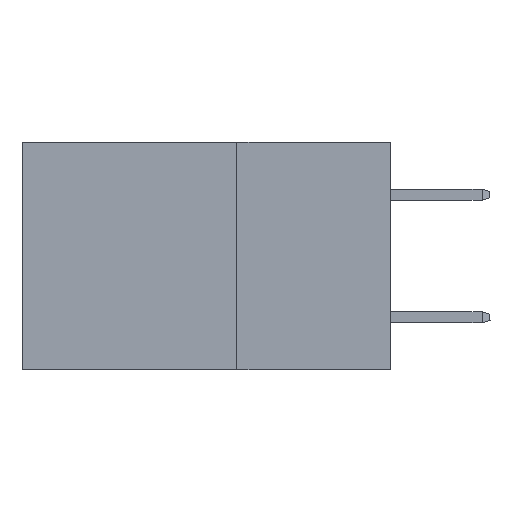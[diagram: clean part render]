
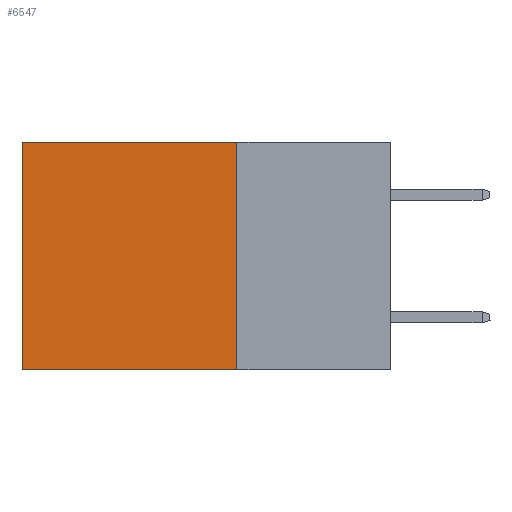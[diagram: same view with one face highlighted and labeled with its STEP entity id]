
A CAD part, left-side view. The second image highlights one B-rep face of the part: STEP entity #6547.
In plain terms, the highlighted planar face has unit normal (-1, 0, 0).
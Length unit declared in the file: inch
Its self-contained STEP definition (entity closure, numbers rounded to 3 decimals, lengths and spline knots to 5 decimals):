
#1896 = ORIENTED_EDGE ( 'NONE', *, *, #3113, .T. ) ;
#1969 = CARTESIAN_POINT ( 'NONE',  ( 0.2875, 0.25, 0. ) ) ;
#3113 = EDGE_CURVE ( 'NONE', #19517, #9737, #12800, .T. ) ;
#5117 = VERTEX_POINT ( 'NONE', #19602 ) ;
#5700 = ORIENTED_EDGE ( 'NONE', *, *, #10846, .F. ) ;
#6547 = ADVANCED_FACE ( 'NONE', ( #13472 ), #15747, .F. ) ;
#7428 = ORIENTED_EDGE ( 'NONE', *, *, #18647, .F. ) ;
#7660 = VECTOR ( 'NONE', #14456, 39.37008 ) ;
#8335 = AXIS2_PLACEMENT_3D ( 'NONE', #1969, #13083, #8481 ) ;
#8481 = DIRECTION ( 'NONE',  ( 0., 0., -1. ) ) ;
#8796 = VERTEX_POINT ( 'NONE', #15431 ) ;
#9110 = ORIENTED_EDGE ( 'NONE', *, *, #13517, .T. ) ;
#9220 = LINE ( 'NONE', #15464, #19022 ) ;
#9481 = CARTESIAN_POINT ( 'NONE',  ( 0.2875, 0.25, 0. ) ) ;
#9737 = VERTEX_POINT ( 'NONE', #13606 ) ;
#9877 = VECTOR ( 'NONE', #21310, 39.37008 ) ;
#10846 = EDGE_CURVE ( 'NONE', #19517, #8796, #18110, .T. ) ;
#12800 = LINE ( 'NONE', #21198, #21281 ) ;
#13083 = DIRECTION ( 'NONE',  ( 1., 0., 0. ) ) ;
#13472 = FACE_OUTER_BOUND ( 'NONE', #15023, .T. ) ;
#13517 = EDGE_CURVE ( 'NONE', #9737, #5117, #9220, .T. ) ;
#13606 = CARTESIAN_POINT ( 'NONE',  ( 0.2875, 0.6, 0. ) ) ;
#14306 = CARTESIAN_POINT ( 'NONE',  ( 0.2875, 0.25, -0.37 ) ) ;
#14392 = CARTESIAN_POINT ( 'NONE',  ( 0.2875, 0.25, 0. ) ) ;
#14456 = DIRECTION ( 'NONE',  ( 0., 1., 0. ) ) ;
#15023 = EDGE_LOOP ( 'NONE', ( #9110, #7428, #5700, #1896 ) ) ;
#15431 = CARTESIAN_POINT ( 'NONE',  ( 0.2875, 0.25, -0.37 ) ) ;
#15464 = CARTESIAN_POINT ( 'NONE',  ( 0.2875, 0.6, 0. ) ) ;
#15747 = PLANE ( 'NONE',  #8335 ) ;
#16150 = DIRECTION ( 'NONE',  ( 0., 1., 0. ) ) ;
#18110 = LINE ( 'NONE', #9481, #9877 ) ;
#18647 = EDGE_CURVE ( 'NONE', #8796, #5117, #20403, .T. ) ;
#18653 = DIRECTION ( 'NONE',  ( 0., 0., -1. ) ) ;
#19022 = VECTOR ( 'NONE', #18653, 39.37008 ) ;
#19517 = VERTEX_POINT ( 'NONE', #14392 ) ;
#19602 = CARTESIAN_POINT ( 'NONE',  ( 0.2875, 0.6, -0.37 ) ) ;
#20403 = LINE ( 'NONE', #14306, #7660 ) ;
#21198 = CARTESIAN_POINT ( 'NONE',  ( 0.2875, 0.25, 0. ) ) ;
#21281 = VECTOR ( 'NONE', #16150, 39.37008 ) ;
#21310 = DIRECTION ( 'NONE',  ( 0., 0., -1. ) ) ;
